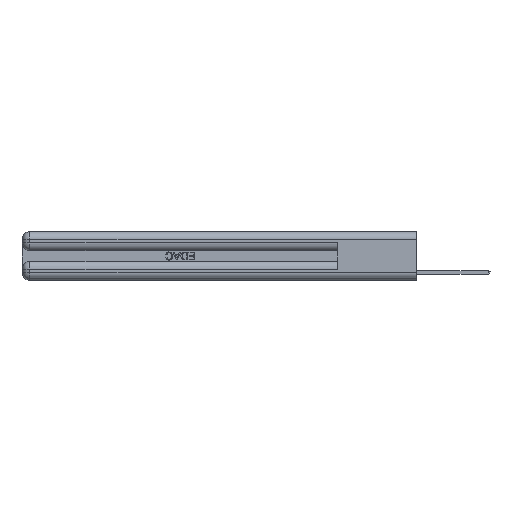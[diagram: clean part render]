
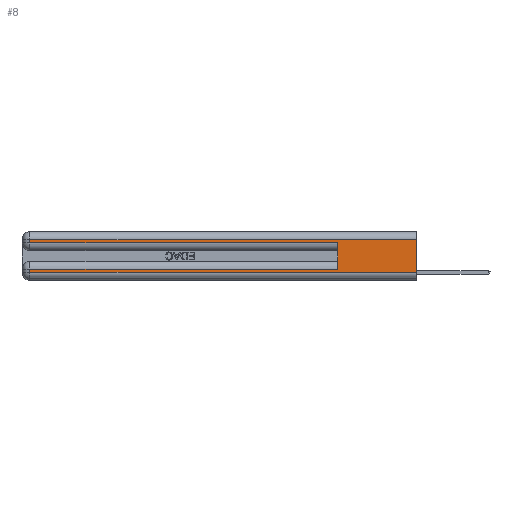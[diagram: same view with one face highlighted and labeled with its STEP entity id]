
A CAD part, left-side view. The second image highlights one B-rep face of the part: STEP entity #8.
In plain terms, the highlighted planar face has unit normal (-1, 0, 0).
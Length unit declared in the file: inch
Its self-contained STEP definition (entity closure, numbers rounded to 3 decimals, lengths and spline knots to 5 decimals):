
#8 = ADVANCED_FACE ( 'NONE', ( #19749 ), #30322, .F. ) ;
#1973 = LINE ( 'NONE', #24791, #9726 ) ;
#3077 = VECTOR ( 'NONE', #13217, 39.37008 ) ;
#3143 = CARTESIAN_POINT ( 'NONE',  ( 0., 2.94, 0.31 ) ) ;
#4406 = EDGE_CURVE ( 'NONE', #12857, #25035, #22741, .T. ) ;
#4826 = LINE ( 'NONE', #12713, #23932 ) ;
#4969 = DIRECTION ( 'NONE',  ( 0., 1., 0. ) ) ;
#6310 = CARTESIAN_POINT ( 'NONE',  ( 0., 0.6, 0.145 ) ) ;
#6975 = DIRECTION ( 'NONE',  ( 0., -1., 0. ) ) ;
#7257 = ORIENTED_EDGE ( 'NONE', *, *, #4406, .T. ) ;
#7376 = EDGE_CURVE ( 'NONE', #32463, #9818, #14242, .T. ) ;
#7398 = LINE ( 'NONE', #17985, #21363 ) ;
#7561 = EDGE_CURVE ( 'NONE', #32463, #25035, #4826, .T. ) ;
#8994 = DIRECTION ( 'NONE',  ( 0., 0., 1. ) ) ;
#9704 = ORIENTED_EDGE ( 'NONE', *, *, #13884, .T. ) ;
#9726 = VECTOR ( 'NONE', #4969, 39.37008 ) ;
#9818 = VERTEX_POINT ( 'NONE', #3143 ) ;
#10027 = VERTEX_POINT ( 'NONE', #32995 ) ;
#10751 = ORIENTED_EDGE ( 'NONE', *, *, #25217, .T. ) ;
#11387 = DIRECTION ( 'NONE',  ( 0., 1., 0. ) ) ;
#11796 = VECTOR ( 'NONE', #11387, 39.37008 ) ;
#12713 = CARTESIAN_POINT ( 'NONE',  ( 0., 0., 0.37 ) ) ;
#12778 = DIRECTION ( 'NONE',  ( 0., -1., 0. ) ) ;
#12857 = VERTEX_POINT ( 'NONE', #25333 ) ;
#13217 = DIRECTION ( 'NONE',  ( 0., 0., -1. ) ) ;
#13816 = CARTESIAN_POINT ( 'NONE',  ( 0., 2.94, 0.37 ) ) ;
#13884 = EDGE_CURVE ( 'NONE', #16946, #29340, #1973, .T. ) ;
#13983 = CARTESIAN_POINT ( 'NONE',  ( 0., 0., 0.06 ) ) ;
#14242 = LINE ( 'NONE', #17271, #11796 ) ;
#15686 = CARTESIAN_POINT ( 'NONE',  ( 0., 0.6, 0.085 ) ) ;
#16507 = DIRECTION ( 'NONE',  ( 0., 0., -1. ) ) ;
#16946 = VERTEX_POINT ( 'NONE', #15686 ) ;
#17271 = CARTESIAN_POINT ( 'NONE',  ( 0., 0., 0.31 ) ) ;
#17498 = ORIENTED_EDGE ( 'NONE', *, *, #7376, .T. ) ;
#17985 = CARTESIAN_POINT ( 'NONE',  ( 0., 0., 0.285 ) ) ;
#18163 = VECTOR ( 'NONE', #16507, 39.37008 ) ;
#18822 = ORIENTED_EDGE ( 'NONE', *, *, #24906, .T. ) ;
#19421 = DIRECTION ( 'NONE',  ( 0., 0., -1. ) ) ;
#19749 = FACE_OUTER_BOUND ( 'NONE', #31899, .T. ) ;
#20056 = CARTESIAN_POINT ( 'NONE',  ( 0., 0., 0.06 ) ) ;
#21258 = CARTESIAN_POINT ( 'NONE',  ( 0., 2.94, 0.37 ) ) ;
#21363 = VECTOR ( 'NONE', #12778, 39.37008 ) ;
#21598 = CARTESIAN_POINT ( 'NONE',  ( 0., 0.6, 0.285 ) ) ;
#21988 = VECTOR ( 'NONE', #6975, 39.37008 ) ;
#22719 = VERTEX_POINT ( 'NONE', #21598 ) ;
#22741 = LINE ( 'NONE', #20056, #21988 ) ;
#22937 = CARTESIAN_POINT ( 'NONE',  ( 0., 2.94, 0.085 ) ) ;
#22940 = DIRECTION ( 'NONE',  ( 0., 0., -1. ) ) ;
#23711 = ORIENTED_EDGE ( 'NONE', *, *, #7561, .F. ) ;
#23932 = VECTOR ( 'NONE', #22940, 39.37008 ) ;
#24791 = CARTESIAN_POINT ( 'NONE',  ( 0., 0., 0.085 ) ) ;
#24906 = EDGE_CURVE ( 'NONE', #29340, #12857, #31764, .T. ) ;
#25035 = VERTEX_POINT ( 'NONE', #13983 ) ;
#25217 = EDGE_CURVE ( 'NONE', #10027, #22719, #7398, .T. ) ;
#25333 = CARTESIAN_POINT ( 'NONE',  ( 0., 2.94, 0.06 ) ) ;
#25754 = AXIS2_PLACEMENT_3D ( 'NONE', #32845, #29994, #19421 ) ;
#28196 = ORIENTED_EDGE ( 'NONE', *, *, #31942, .T. ) ;
#29315 = LINE ( 'NONE', #6310, #30952 ) ;
#29340 = VERTEX_POINT ( 'NONE', #22937 ) ;
#29521 = ORIENTED_EDGE ( 'NONE', *, *, #32189, .F. ) ;
#29994 = DIRECTION ( 'NONE',  ( 1., 0., 0. ) ) ;
#30322 = PLANE ( 'NONE',  #25754 ) ;
#30952 = VECTOR ( 'NONE', #8994, 39.37008 ) ;
#31670 = LINE ( 'NONE', #21258, #3077 ) ;
#31764 = LINE ( 'NONE', #13816, #18163 ) ;
#31899 = EDGE_LOOP ( 'NONE', ( #23711, #17498, #28196, #10751, #29521, #9704, #18822, #7257 ) ) ;
#31942 = EDGE_CURVE ( 'NONE', #9818, #10027, #31670, .T. ) ;
#32128 = CARTESIAN_POINT ( 'NONE',  ( 0., 0., 0.31 ) ) ;
#32189 = EDGE_CURVE ( 'NONE', #16946, #22719, #29315, .T. ) ;
#32463 = VERTEX_POINT ( 'NONE', #32128 ) ;
#32845 = CARTESIAN_POINT ( 'NONE',  ( 0., 0., 0.37 ) ) ;
#32995 = CARTESIAN_POINT ( 'NONE',  ( 0., 2.94, 0.285 ) ) ;
